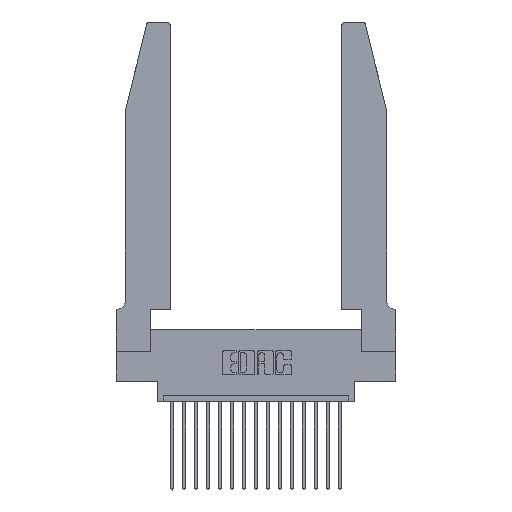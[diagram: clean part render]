
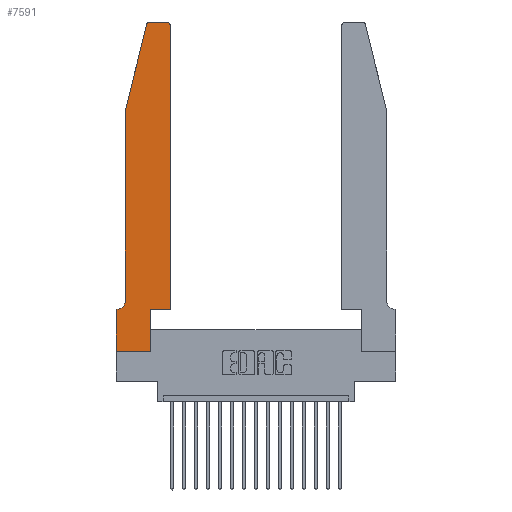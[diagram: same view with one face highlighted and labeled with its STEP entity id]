
A CAD part, top view. The second image highlights one B-rep face of the part: STEP entity #7591.
In plain terms, the highlighted planar face has unit normal (0, 0, 1).
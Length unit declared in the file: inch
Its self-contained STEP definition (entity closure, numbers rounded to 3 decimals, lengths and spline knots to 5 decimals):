
#161 = LINE ( 'NONE', #3540, #2810 ) ;
#187 = CARTESIAN_POINT ( 'NONE',  ( 0.4505, 0.35, 0.37 ) ) ;
#396 = ORIENTED_EDGE ( 'NONE', *, *, #2972, .T. ) ;
#958 = VECTOR ( 'NONE', #19668, 39.37008 ) ;
#1085 = CARTESIAN_POINT ( 'NONE',  ( 0.4505, 2.72, 0.37 ) ) ;
#1351 = DIRECTION ( 'NONE',  ( -0.239, -0.971, 0. ) ) ;
#1422 = CARTESIAN_POINT ( 'NONE',  ( 0., 0.35, 0.37 ) ) ;
#1724 = ORIENTED_EDGE ( 'NONE', *, *, #11098, .T. ) ;
#2171 = CARTESIAN_POINT ( 'NONE',  ( 0.284, 2.72, 0.37 ) ) ;
#2379 = VECTOR ( 'NONE', #5592, 39.37008 ) ;
#2566 = LINE ( 'NONE', #187, #3547 ) ;
#2810 = VECTOR ( 'NONE', #11027, 39.37008 ) ;
#2972 = EDGE_CURVE ( 'NONE', #5320, #15921, #8121, .T. ) ;
#3074 = EDGE_CURVE ( 'NONE', #19836, #18856, #4989, .T. ) ;
#3101 = AXIS2_PLACEMENT_3D ( 'NONE', #2171, #13007, #14552 ) ;
#3301 = ORIENTED_EDGE ( 'NONE', *, *, #5424, .T. ) ;
#3540 = CARTESIAN_POINT ( 'NONE',  ( 0., 0., 0.37 ) ) ;
#3547 = VECTOR ( 'NONE', #12451, 39.37008 ) ;
#4225 = EDGE_CURVE ( 'NONE', #19575, #8133, #2566, .T. ) ;
#4549 = CARTESIAN_POINT ( 'NONE',  ( 0.0755, 0.42, 0.37 ) ) ;
#4789 = LINE ( 'NONE', #16591, #11294 ) ;
#4830 = CARTESIAN_POINT ( 'NONE',  ( 0.0755, 0.35, 0.37 ) ) ;
#4989 = LINE ( 'NONE', #19558, #2379 ) ;
#5288 = CARTESIAN_POINT ( 'NONE',  ( 0., 0.35, 0.37 ) ) ;
#5320 = VERTEX_POINT ( 'NONE', #8655 ) ;
#5424 = EDGE_CURVE ( 'NONE', #8133, #16356, #13068, .T. ) ;
#5592 = DIRECTION ( 'NONE',  ( 0., -1., 0. ) ) ;
#5626 = DIRECTION ( 'NONE',  ( 0., 0., -1. ) ) ;
#5763 = CARTESIAN_POINT ( 'NONE',  ( 0.0755, 2., 0.37 ) ) ;
#5770 = DIRECTION ( 'NONE',  ( 0., 0., 1. ) ) ;
#5951 = AXIS2_PLACEMENT_3D ( 'NONE', #11815, #5770, #15012 ) ;
#6179 = VECTOR ( 'NONE', #8750, 39.37008 ) ;
#6552 = CARTESIAN_POINT ( 'NONE',  ( 0.2865, 0.35, 0.37 ) ) ;
#7218 = VERTEX_POINT ( 'NONE', #7639 ) ;
#7230 = ORIENTED_EDGE ( 'NONE', *, *, #15175, .T. ) ;
#7509 = EDGE_CURVE ( 'NONE', #7218, #11544, #7739, .T. ) ;
#7591 = ADVANCED_FACE ( 'NONE', ( #13488 ), #11992, .T. ) ;
#7639 = CARTESIAN_POINT ( 'NONE',  ( 0.284, 2.75, 0.37 ) ) ;
#7739 = CIRCLE ( 'NONE', #3101, 0.03 ) ;
#7917 = DIRECTION ( 'NONE',  ( -1., 0., 0. ) ) ;
#8121 = LINE ( 'NONE', #4830, #16736 ) ;
#8133 = VERTEX_POINT ( 'NONE', #1085 ) ;
#8655 = CARTESIAN_POINT ( 'NONE',  ( 0.0055, 0.35, 0.37 ) ) ;
#8750 = DIRECTION ( 'NONE',  ( -1., 0., 0. ) ) ;
#8822 = ORIENTED_EDGE ( 'NONE', *, *, #16091, .T. ) ;
#8987 = ORIENTED_EDGE ( 'NONE', *, *, #11603, .T. ) ;
#9079 = ORIENTED_EDGE ( 'NONE', *, *, #9210, .T. ) ;
#9095 = AXIS2_PLACEMENT_3D ( 'NONE', #11732, #5626, #16327 ) ;
#9115 = EDGE_CURVE ( 'NONE', #11544, #19836, #4789, .T. ) ;
#9210 = EDGE_CURVE ( 'NONE', #11412, #15585, #18683, .T. ) ;
#9760 = VECTOR ( 'NONE', #15164, 39.37008 ) ;
#10199 = ORIENTED_EDGE ( 'NONE', *, *, #7509, .T. ) ;
#11027 = DIRECTION ( 'NONE',  ( 0., -1., 0. ) ) ;
#11098 = EDGE_CURVE ( 'NONE', #15585, #18921, #11719, .T. ) ;
#11294 = VECTOR ( 'NONE', #1351, 39.37008 ) ;
#11309 = AXIS2_PLACEMENT_3D ( 'NONE', #1422, #15275, #13460 ) ;
#11412 = VERTEX_POINT ( 'NONE', #17499 ) ;
#11544 = VERTEX_POINT ( 'NONE', #12053 ) ;
#11603 = EDGE_CURVE ( 'NONE', #18921, #19575, #14337, .T. ) ;
#11719 = LINE ( 'NONE', #18602, #15042 ) ;
#11732 = CARTESIAN_POINT ( 'NONE',  ( 0.0055, 0.42, 0.37 ) ) ;
#11815 = CARTESIAN_POINT ( 'NONE',  ( 0.4205, 2.72, 0.37 ) ) ;
#11992 = PLANE ( 'NONE',  #11309 ) ;
#12053 = CARTESIAN_POINT ( 'NONE',  ( 0.25487, 2.72718, 0.37 ) ) ;
#12382 = CARTESIAN_POINT ( 'NONE',  ( 0.4205, 2.75, 0.37 ) ) ;
#12451 = DIRECTION ( 'NONE',  ( 0., 1., 0. ) ) ;
#12853 = ORIENTED_EDGE ( 'NONE', *, *, #3074, .T. ) ;
#13007 = DIRECTION ( 'NONE',  ( 0., 0., 1. ) ) ;
#13068 = CIRCLE ( 'NONE', #5951, 0.03 ) ;
#13216 = CARTESIAN_POINT ( 'NONE',  ( 0.4505, 0.35, 0.37 ) ) ;
#13460 = DIRECTION ( 'NONE',  ( 1., 0., 0. ) ) ;
#13463 = CARTESIAN_POINT ( 'NONE',  ( 0., 0., 0.37 ) ) ;
#13488 = FACE_OUTER_BOUND ( 'NONE', #18130, .T. ) ;
#14337 = LINE ( 'NONE', #16622, #9760 ) ;
#14552 = DIRECTION ( 'NONE',  ( 1., 0., 0. ) ) ;
#14884 = ORIENTED_EDGE ( 'NONE', *, *, #4225, .T. ) ;
#14927 = EDGE_CURVE ( 'NONE', #16356, #7218, #19334, .T. ) ;
#15012 = DIRECTION ( 'NONE',  ( 1., 0., 0. ) ) ;
#15042 = VECTOR ( 'NONE', #17168, 39.37008 ) ;
#15164 = DIRECTION ( 'NONE',  ( 1., 0., 0. ) ) ;
#15175 = EDGE_CURVE ( 'NONE', #15921, #11412, #161, .T. ) ;
#15275 = DIRECTION ( 'NONE',  ( 0., 0., 1. ) ) ;
#15316 = ORIENTED_EDGE ( 'NONE', *, *, #9115, .T. ) ;
#15585 = VERTEX_POINT ( 'NONE', #19756 ) ;
#15921 = VERTEX_POINT ( 'NONE', #5288 ) ;
#16091 = EDGE_CURVE ( 'NONE', #18856, #5320, #18083, .T. ) ;
#16327 = DIRECTION ( 'NONE',  ( -1., 0., 0. ) ) ;
#16356 = VERTEX_POINT ( 'NONE', #12382 ) ;
#16516 = ORIENTED_EDGE ( 'NONE', *, *, #14927, .T. ) ;
#16591 = CARTESIAN_POINT ( 'NONE',  ( 0.0755, 2., 0.37 ) ) ;
#16622 = CARTESIAN_POINT ( 'NONE',  ( 0.4505, 0.35, 0.37 ) ) ;
#16736 = VECTOR ( 'NONE', #7917, 39.37008 ) ;
#17168 = DIRECTION ( 'NONE',  ( 0., 1., 0. ) ) ;
#17499 = CARTESIAN_POINT ( 'NONE',  ( 0., 0., 0.37 ) ) ;
#18036 = CARTESIAN_POINT ( 'NONE',  ( 0.2605, 2.75, 0.37 ) ) ;
#18083 = CIRCLE ( 'NONE', #9095, 0.07 ) ;
#18130 = EDGE_LOOP ( 'NONE', ( #16516, #10199, #15316, #12853, #8822, #396, #7230, #9079, #1724, #8987, #14884, #3301 ) ) ;
#18602 = CARTESIAN_POINT ( 'NONE',  ( 0.2865, 0.35, 0.37 ) ) ;
#18683 = LINE ( 'NONE', #13463, #958 ) ;
#18856 = VERTEX_POINT ( 'NONE', #4549 ) ;
#18921 = VERTEX_POINT ( 'NONE', #6552 ) ;
#19334 = LINE ( 'NONE', #18036, #6179 ) ;
#19558 = CARTESIAN_POINT ( 'NONE',  ( 0.0755, 2., 0.37 ) ) ;
#19575 = VERTEX_POINT ( 'NONE', #13216 ) ;
#19668 = DIRECTION ( 'NONE',  ( 1., 0., 0. ) ) ;
#19756 = CARTESIAN_POINT ( 'NONE',  ( 0.2865, 0., 0.37 ) ) ;
#19836 = VERTEX_POINT ( 'NONE', #5763 ) ;
